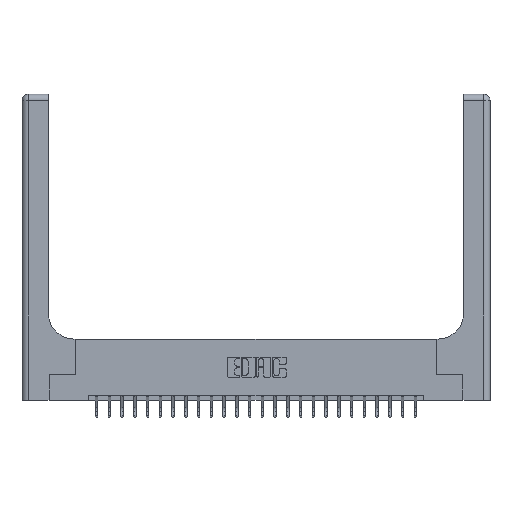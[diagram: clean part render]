
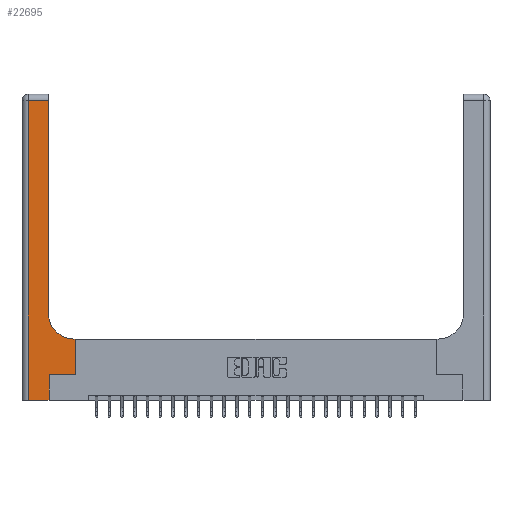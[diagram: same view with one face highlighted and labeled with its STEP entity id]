
A CAD part, top view. The second image highlights one B-rep face of the part: STEP entity #22695.
In plain terms, the highlighted planar face has unit normal (0, 0, 1).
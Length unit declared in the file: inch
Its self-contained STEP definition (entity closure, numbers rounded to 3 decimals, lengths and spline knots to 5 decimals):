
#148 = EDGE_CURVE ( 'NONE', #21384, #14509, #5001, .T. ) ;
#265 = VECTOR ( 'NONE', #1069, 39.37008 ) ;
#696 = LINE ( 'NONE', #6515, #1367 ) ;
#839 = ORIENTED_EDGE ( 'NONE', *, *, #9326, .T. ) ;
#1050 = CARTESIAN_POINT ( 'NONE',  ( 0.51, 0.6, 0.37 ) ) ;
#1069 = DIRECTION ( 'NONE',  ( 0., 1., 0. ) ) ;
#1300 = CARTESIAN_POINT ( 'NONE',  ( 0.06, 3., 0.37 ) ) ;
#1367 = VECTOR ( 'NONE', #21933, 39.37008 ) ;
#1898 = ORIENTED_EDGE ( 'NONE', *, *, #148, .T. ) ;
#2100 = EDGE_CURVE ( 'NONE', #15843, #14256, #16572, .T. ) ;
#2570 = CARTESIAN_POINT ( 'NONE',  ( 0.265, 0., 0.37 ) ) ;
#3184 = VERTEX_POINT ( 'NONE', #2570 ) ;
#4332 = CARTESIAN_POINT ( 'NONE',  ( 0.528, 0.6, 0.37 ) ) ;
#5001 = LINE ( 'NONE', #6511, #23806 ) ;
#5451 = EDGE_CURVE ( 'NONE', #20035, #15843, #696, .T. ) ;
#5965 = CARTESIAN_POINT ( 'NONE',  ( 0.528, 0.25, 0.37 ) ) ;
#6434 = EDGE_CURVE ( 'NONE', #11918, #3184, #9818, .T. ) ;
#6498 = DIRECTION ( 'NONE',  ( 1., 0., 0. ) ) ;
#6511 = CARTESIAN_POINT ( 'NONE',  ( 0., 2.94, 0.37 ) ) ;
#6515 = CARTESIAN_POINT ( 'NONE',  ( 0.26, 0.6, 0.37 ) ) ;
#6659 = VECTOR ( 'NONE', #10372, 39.37008 ) ;
#7102 = VECTOR ( 'NONE', #6498, 39.37008 ) ;
#7234 = EDGE_CURVE ( 'NONE', #14509, #11918, #20265, .T. ) ;
#7846 = LINE ( 'NONE', #16956, #6659 ) ;
#8066 = ORIENTED_EDGE ( 'NONE', *, *, #24217, .T. ) ;
#8258 = DIRECTION ( 'NONE',  ( 0., 1., 0. ) ) ;
#8543 = EDGE_CURVE ( 'NONE', #14412, #21312, #23568, .T. ) ;
#8548 = DIRECTION ( 'NONE',  ( -1., 0., 0. ) ) ;
#8657 = VECTOR ( 'NONE', #24442, 39.37008 ) ;
#9326 = EDGE_CURVE ( 'NONE', #3184, #14412, #7846, .T. ) ;
#9703 = AXIS2_PLACEMENT_3D ( 'NONE', #20627, #24551, #11536 ) ;
#9818 = LINE ( 'NONE', #22251, #17169 ) ;
#9876 = CARTESIAN_POINT ( 'NONE',  ( 0.26, 0.85, 0.37 ) ) ;
#10372 = DIRECTION ( 'NONE',  ( 0., 1., 0. ) ) ;
#10842 = ORIENTED_EDGE ( 'NONE', *, *, #2100, .T. ) ;
#10931 = AXIS2_PLACEMENT_3D ( 'NONE', #18483, #22630, #11028 ) ;
#11028 = DIRECTION ( 'NONE',  ( -1., 0., 0. ) ) ;
#11536 = DIRECTION ( 'NONE',  ( 1., 0., 0. ) ) ;
#11751 = EDGE_CURVE ( 'NONE', #21312, #20035, #22166, .T. ) ;
#11918 = VERTEX_POINT ( 'NONE', #13236 ) ;
#11920 = CARTESIAN_POINT ( 'NONE',  ( 0.26, 3., 0.37 ) ) ;
#12043 = LINE ( 'NONE', #11920, #24622 ) ;
#12672 = CARTESIAN_POINT ( 'NONE',  ( 0.26, 2.94, 0.37 ) ) ;
#13030 = CARTESIAN_POINT ( 'NONE',  ( 0.06, 2.94, 0.37 ) ) ;
#13236 = CARTESIAN_POINT ( 'NONE',  ( 0.06, 0., 0.37 ) ) ;
#13249 = DIRECTION ( 'NONE',  ( 1., 0., 0. ) ) ;
#14232 = CARTESIAN_POINT ( 'NONE',  ( 0.528, 0.25, 0.37 ) ) ;
#14256 = VERTEX_POINT ( 'NONE', #9876 ) ;
#14412 = VERTEX_POINT ( 'NONE', #19986 ) ;
#14509 = VERTEX_POINT ( 'NONE', #13030 ) ;
#14638 = ORIENTED_EDGE ( 'NONE', *, *, #8543, .T. ) ;
#14945 = PLANE ( 'NONE',  #10931 ) ;
#15398 = ORIENTED_EDGE ( 'NONE', *, *, #6434, .T. ) ;
#15843 = VERTEX_POINT ( 'NONE', #1050 ) ;
#16428 = ORIENTED_EDGE ( 'NONE', *, *, #5451, .T. ) ;
#16572 = CIRCLE ( 'NONE', #9703, 0.25 ) ;
#16956 = CARTESIAN_POINT ( 'NONE',  ( 0.265, 0., 0.37 ) ) ;
#17169 = VECTOR ( 'NONE', #13249, 39.37008 ) ;
#18131 = CARTESIAN_POINT ( 'NONE',  ( 0.265, 0.25, 0.37 ) ) ;
#18483 = CARTESIAN_POINT ( 'NONE',  ( 0., 3., 0.37 ) ) ;
#18678 = ORIENTED_EDGE ( 'NONE', *, *, #11751, .T. ) ;
#19986 = CARTESIAN_POINT ( 'NONE',  ( 0.265, 0.25, 0.37 ) ) ;
#20035 = VERTEX_POINT ( 'NONE', #4332 ) ;
#20265 = LINE ( 'NONE', #1300, #8657 ) ;
#20627 = CARTESIAN_POINT ( 'NONE',  ( 0.51, 0.85, 0.37 ) ) ;
#21312 = VERTEX_POINT ( 'NONE', #5965 ) ;
#21384 = VERTEX_POINT ( 'NONE', #12672 ) ;
#21933 = DIRECTION ( 'NONE',  ( -1., 0., 0. ) ) ;
#22166 = LINE ( 'NONE', #14232, #265 ) ;
#22251 = CARTESIAN_POINT ( 'NONE',  ( 0., 0., 0.37 ) ) ;
#22630 = DIRECTION ( 'NONE',  ( 0., 0., -1. ) ) ;
#22695 = ADVANCED_FACE ( 'NONE', ( #24165 ), #14945, .F. ) ;
#23263 = ORIENTED_EDGE ( 'NONE', *, *, #7234, .T. ) ;
#23568 = LINE ( 'NONE', #18131, #7102 ) ;
#23806 = VECTOR ( 'NONE', #8548, 39.37008 ) ;
#24165 = FACE_OUTER_BOUND ( 'NONE', #24193, .T. ) ;
#24193 = EDGE_LOOP ( 'NONE', ( #8066, #1898, #23263, #15398, #839, #14638, #18678, #16428, #10842 ) ) ;
#24217 = EDGE_CURVE ( 'NONE', #14256, #21384, #12043, .T. ) ;
#24442 = DIRECTION ( 'NONE',  ( 0., -1., 0. ) ) ;
#24551 = DIRECTION ( 'NONE',  ( 0., 0., -1. ) ) ;
#24622 = VECTOR ( 'NONE', #8258, 39.37008 ) ;
